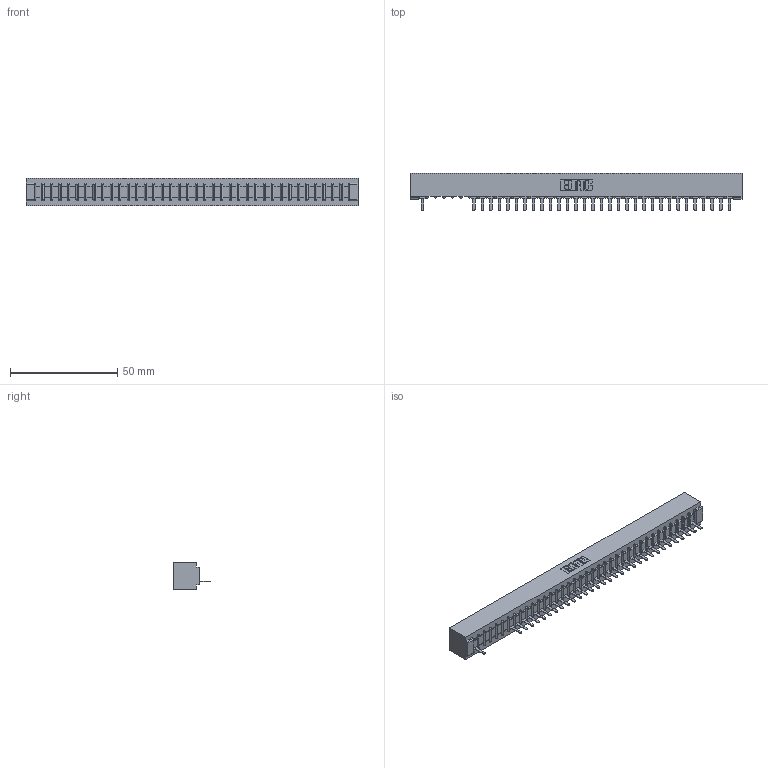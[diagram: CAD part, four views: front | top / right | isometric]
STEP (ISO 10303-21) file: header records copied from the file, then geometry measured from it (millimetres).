
FILE_DESCRIPTION (( 'STEP AP203' ), '1' );
FILE_NAME ('357-037-521-101.STEP', '2018-08-10T07:46:51', ( '' ), ( '' ), 'SwSTEP 2.0', 'SolidWorks 2016', '' );
FILE_SCHEMA (( 'CONFIG_CONTROL_DESIGN' ));
Length unit declared in the file: inch
Products named in the file (3): 307 Part_No Mounting Lugs; 307-290-002_521; 357-037-521-101
Assembly tree (33 placements, depth 2):
  357-037-521-101
    307 Part_No Mounting Lugs
    307-290-002_521  x32
Bounding box: 154.48 x 17.42 x 12.7 mm (x, y, z)
Volume: 16909.3 mm3; surface area: 20579.7 mm2
Topology: 33 solids, 33 shells, 2616 faces, 8043 edges, 5258 vertices
Faces by surface type: plane 1566, cylinder 974, sphere 76
Entity records: 32616 total; most frequent: CARTESIAN_POINT 5523, ORIENTED_EDGE 5518, DIRECTION 5361, EDGE_CURVE 2759, VECTOR 2113, LINE 2113, VERTEX_POINT 1786, AXIS2_PLACEMENT_3D 1624
